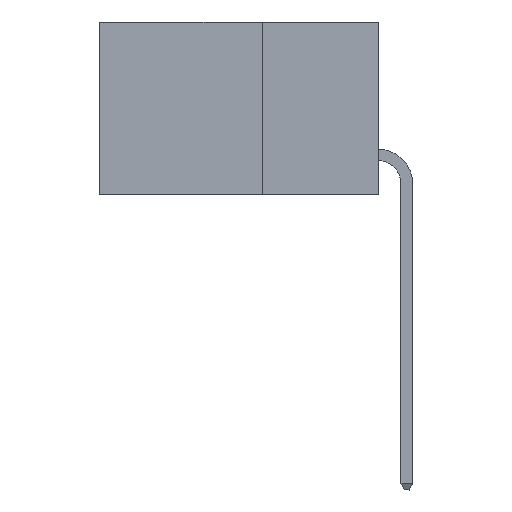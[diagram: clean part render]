
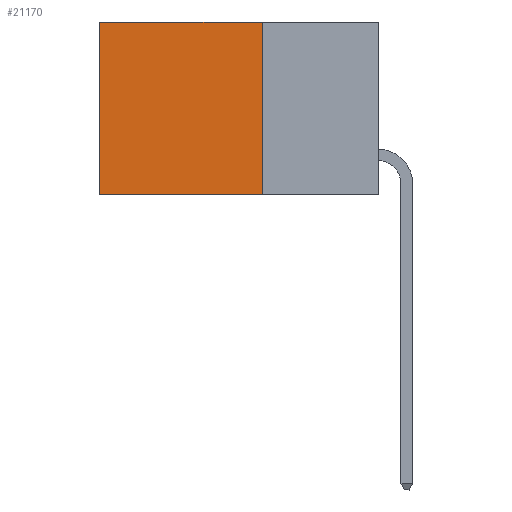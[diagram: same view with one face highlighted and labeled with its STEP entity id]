
A CAD part, left-side view. The second image highlights one B-rep face of the part: STEP entity #21170.
In plain terms, the highlighted planar face has unit normal (-1, 0, 0).
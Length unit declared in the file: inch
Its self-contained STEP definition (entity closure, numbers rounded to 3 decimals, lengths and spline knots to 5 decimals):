
#325 = CARTESIAN_POINT ( 'NONE',  ( 0.298, 0.25, -0.37 ) ) ;
#395 = VECTOR ( 'NONE', #15469, 39.37008 ) ;
#1289 = DIRECTION ( 'NONE',  ( 0., 1., 0. ) ) ;
#1797 = EDGE_CURVE ( 'NONE', #8366, #15729, #18729, .T. ) ;
#1854 = CARTESIAN_POINT ( 'NONE',  ( 0.298, 0.25, 0. ) ) ;
#2060 = VECTOR ( 'NONE', #10569, 39.37008 ) ;
#2587 = LINE ( 'NONE', #1854, #2060 ) ;
#2663 = ORIENTED_EDGE ( 'NONE', *, *, #9314, .F. ) ;
#4364 = VERTEX_POINT ( 'NONE', #15517 ) ;
#4943 = ORIENTED_EDGE ( 'NONE', *, *, #1797, .T. ) ;
#5797 = CARTESIAN_POINT ( 'NONE',  ( 0.298, 0.25, 0. ) ) ;
#7562 = DIRECTION ( 'NONE',  ( 1., 0., 0. ) ) ;
#7564 = ORIENTED_EDGE ( 'NONE', *, *, #8552, .F. ) ;
#8366 = VERTEX_POINT ( 'NONE', #11522 ) ;
#8552 = EDGE_CURVE ( 'NONE', #13500, #15729, #19010, .T. ) ;
#8752 = VECTOR ( 'NONE', #1289, 39.37008 ) ;
#9295 = LINE ( 'NONE', #22198, #8752 ) ;
#9314 = EDGE_CURVE ( 'NONE', #4364, #13500, #2587, .T. ) ;
#10569 = DIRECTION ( 'NONE',  ( 0., 0., -1. ) ) ;
#11067 = ORIENTED_EDGE ( 'NONE', *, *, #17804, .T. ) ;
#11522 = CARTESIAN_POINT ( 'NONE',  ( 0.298, 0.6, 0. ) ) ;
#13500 = VERTEX_POINT ( 'NONE', #325 ) ;
#13737 = CARTESIAN_POINT ( 'NONE',  ( 0.298, 0.25, -0.37 ) ) ;
#14116 = VECTOR ( 'NONE', #22215, 39.37008 ) ;
#15422 = CARTESIAN_POINT ( 'NONE',  ( 0.298, 0.6, -0.37 ) ) ;
#15469 = DIRECTION ( 'NONE',  ( 0., 1., 0. ) ) ;
#15517 = CARTESIAN_POINT ( 'NONE',  ( 0.298, 0.25, 0. ) ) ;
#15729 = VERTEX_POINT ( 'NONE', #15422 ) ;
#16242 = PLANE ( 'NONE',  #20925 ) ;
#17157 = FACE_OUTER_BOUND ( 'NONE', #17562, .T. ) ;
#17562 = EDGE_LOOP ( 'NONE', ( #4943, #7564, #2663, #11067 ) ) ;
#17804 = EDGE_CURVE ( 'NONE', #4364, #8366, #9295, .T. ) ;
#18729 = LINE ( 'NONE', #22090, #14116 ) ;
#19010 = LINE ( 'NONE', #13737, #395 ) ;
#19736 = DIRECTION ( 'NONE',  ( 0., 0., -1. ) ) ;
#20925 = AXIS2_PLACEMENT_3D ( 'NONE', #5797, #7562, #19736 ) ;
#21170 = ADVANCED_FACE ( 'NONE', ( #17157 ), #16242, .F. ) ;
#22090 = CARTESIAN_POINT ( 'NONE',  ( 0.298, 0.6, 0. ) ) ;
#22198 = CARTESIAN_POINT ( 'NONE',  ( 0.298, 0.25, 0. ) ) ;
#22215 = DIRECTION ( 'NONE',  ( 0., 0., -1. ) ) ;
